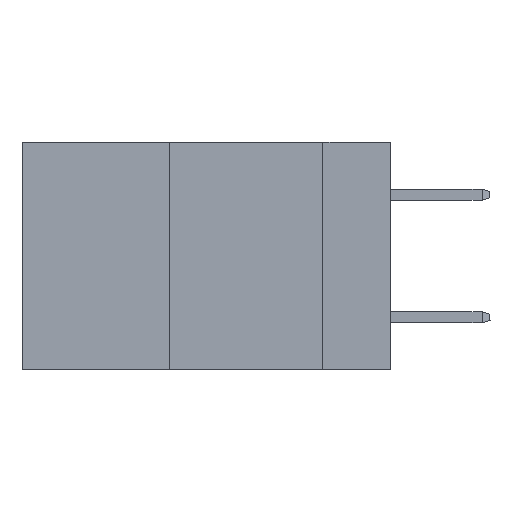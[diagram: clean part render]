
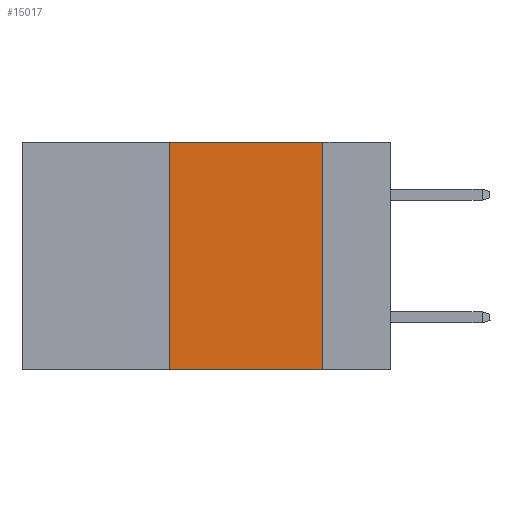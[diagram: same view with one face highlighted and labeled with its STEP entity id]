
A CAD part, left-side view. The second image highlights one B-rep face of the part: STEP entity #15017.
In plain terms, the highlighted planar face has unit normal (-1, 0, 0).
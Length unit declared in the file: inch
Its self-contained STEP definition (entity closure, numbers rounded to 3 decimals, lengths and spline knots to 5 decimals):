
#1055 = CARTESIAN_POINT ( 'NONE',  ( 0., 0.6, 0. ) ) ;
#9785 = CARTESIAN_POINT ( 'NONE',  ( 0., 0.6, -0.37 ) ) ;
#9960 = ORIENTED_EDGE ( 'NONE', *, *, #26389, .F. ) ;
#10113 = VERTEX_POINT ( 'NONE', #12605 ) ;
#10354 = VECTOR ( 'NONE', #42127, 39.37008 ) ;
#10504 = ORIENTED_EDGE ( 'NONE', *, *, #43889, .F. ) ;
#12605 = CARTESIAN_POINT ( 'NONE',  ( 0., 0.11, -0.37 ) ) ;
#13332 = DIRECTION ( 'NONE',  ( 0., -1., 0. ) ) ;
#13851 = CARTESIAN_POINT ( 'NONE',  ( 0., 0.36, 0. ) ) ;
#14285 = VECTOR ( 'NONE', #22205, 39.37008 ) ;
#15017 = ADVANCED_FACE ( 'NONE', ( #44953 ), #36616, .F. ) ;
#15756 = DIRECTION ( 'NONE',  ( 1., 0., 0. ) ) ;
#17239 = VERTEX_POINT ( 'NONE', #24904 ) ;
#17364 = VECTOR ( 'NONE', #20115, 39.37008 ) ;
#17565 = CARTESIAN_POINT ( 'NONE',  ( 0., 0.11, 0. ) ) ;
#18543 = LINE ( 'NONE', #31625, #10354 ) ;
#18670 = ORIENTED_EDGE ( 'NONE', *, *, #19202, .F. ) ;
#19202 = EDGE_CURVE ( 'NONE', #28555, #10113, #35854, .T. ) ;
#19282 = ORIENTED_EDGE ( 'NONE', *, *, #32436, .T. ) ;
#19971 = CARTESIAN_POINT ( 'NONE',  ( 0., 0.11, 0. ) ) ;
#20115 = DIRECTION ( 'NONE',  ( 0., 0., -1. ) ) ;
#22037 = LINE ( 'NONE', #9785, #31313 ) ;
#22205 = DIRECTION ( 'NONE',  ( 0., -1., 0. ) ) ;
#24904 = CARTESIAN_POINT ( 'NONE',  ( 0., 0.36, -0.37 ) ) ;
#26389 = EDGE_CURVE ( 'NONE', #34902, #28555, #42027, .T. ) ;
#28261 = EDGE_LOOP ( 'NONE', ( #18670, #9960, #10504, #19282 ) ) ;
#28555 = VERTEX_POINT ( 'NONE', #17565 ) ;
#31313 = VECTOR ( 'NONE', #13332, 39.37008 ) ;
#31625 = CARTESIAN_POINT ( 'NONE',  ( 0., 0.36, 0. ) ) ;
#32436 = EDGE_CURVE ( 'NONE', #17239, #10113, #22037, .T. ) ;
#34419 = AXIS2_PLACEMENT_3D ( 'NONE', #43430, #15756, #40106 ) ;
#34902 = VERTEX_POINT ( 'NONE', #13851 ) ;
#35854 = LINE ( 'NONE', #19971, #17364 ) ;
#36616 = PLANE ( 'NONE',  #34419 ) ;
#40106 = DIRECTION ( 'NONE',  ( 0., 0., -1. ) ) ;
#42027 = LINE ( 'NONE', #1055, #14285 ) ;
#42127 = DIRECTION ( 'NONE',  ( 0., 0., 1. ) ) ;
#43430 = CARTESIAN_POINT ( 'NONE',  ( 0., 0.6, 0. ) ) ;
#43889 = EDGE_CURVE ( 'NONE', #17239, #34902, #18543, .T. ) ;
#44953 = FACE_OUTER_BOUND ( 'NONE', #28261, .T. ) ;
